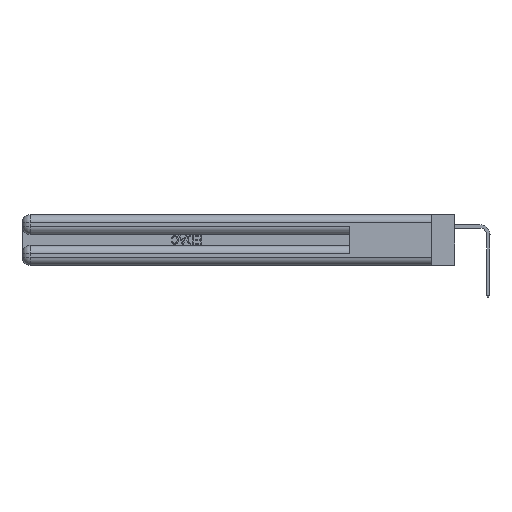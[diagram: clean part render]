
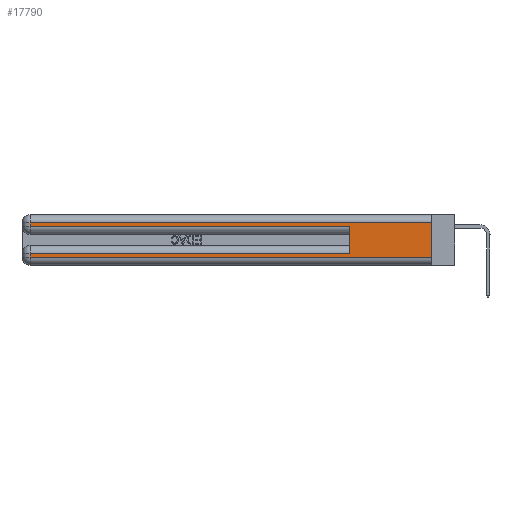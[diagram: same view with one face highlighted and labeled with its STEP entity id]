
A CAD part, left-side view. The second image highlights one B-rep face of the part: STEP entity #17790.
In plain terms, the highlighted planar face has unit normal (-1, 0, 0).
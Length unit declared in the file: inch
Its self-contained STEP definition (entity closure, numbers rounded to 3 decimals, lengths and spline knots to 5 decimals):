
#31 = DIRECTION ( 'NONE',  ( 0., 0., -1. ) ) ;
#1540 = ORIENTED_EDGE ( 'NONE', *, *, #18383, .T. ) ;
#2909 = EDGE_CURVE ( 'NONE', #14189, #25815, #42694, .T. ) ;
#3373 = DIRECTION ( 'NONE',  ( 0., 0., -1. ) ) ;
#3697 = VECTOR ( 'NONE', #49664, 39.37008 ) ;
#3704 = VECTOR ( 'NONE', #16818, 39.37008 ) ;
#4127 = EDGE_CURVE ( 'NONE', #10001, #32581, #5407, .T. ) ;
#4597 = VERTEX_POINT ( 'NONE', #41299 ) ;
#5407 = LINE ( 'NONE', #25441, #39247 ) ;
#7074 = DIRECTION ( 'NONE',  ( 0., 1., 0. ) ) ;
#7449 = CARTESIAN_POINT ( 'NONE',  ( 0., 0.6, 0.145 ) ) ;
#10001 = VERTEX_POINT ( 'NONE', #15341 ) ;
#10906 = EDGE_LOOP ( 'NONE', ( #52240, #1540, #43547, #44859, #22617, #43677, #44469, #35315 ) ) ;
#11749 = CARTESIAN_POINT ( 'NONE',  ( 0., 2.94, 0.285 ) ) ;
#14189 = VERTEX_POINT ( 'NONE', #26636 ) ;
#14384 = LINE ( 'NONE', #15727, #23009 ) ;
#15008 = LINE ( 'NONE', #36868, #3697 ) ;
#15341 = CARTESIAN_POINT ( 'NONE',  ( 0., 2.94, 0.31 ) ) ;
#15727 = CARTESIAN_POINT ( 'NONE',  ( 0., 2.94, 0.37 ) ) ;
#16026 = DIRECTION ( 'NONE',  ( 0., 0., 1. ) ) ;
#16818 = DIRECTION ( 'NONE',  ( 0., 0., -1. ) ) ;
#17790 = ADVANCED_FACE ( 'NONE', ( #39745 ), #54167, .F. ) ;
#18383 = EDGE_CURVE ( 'NONE', #41855, #10001, #15008, .T. ) ;
#19090 = CARTESIAN_POINT ( 'NONE',  ( 0., 0., 0.285 ) ) ;
#19695 = CARTESIAN_POINT ( 'NONE',  ( 0., 0.6, 0.085 ) ) ;
#19762 = VERTEX_POINT ( 'NONE', #19695 ) ;
#20041 = LINE ( 'NONE', #32479, #42573 ) ;
#20544 = VECTOR ( 'NONE', #48741, 39.37008 ) ;
#20728 = CARTESIAN_POINT ( 'NONE',  ( 0., 0., 0.06 ) ) ;
#22617 = ORIENTED_EDGE ( 'NONE', *, *, #54574, .F. ) ;
#23009 = VECTOR ( 'NONE', #49634, 39.37008 ) ;
#25441 = CARTESIAN_POINT ( 'NONE',  ( 0., 2.94, 0.37 ) ) ;
#25679 = EDGE_CURVE ( 'NONE', #50359, #14189, #14384, .T. ) ;
#25815 = VERTEX_POINT ( 'NONE', #20728 ) ;
#25864 = EDGE_CURVE ( 'NONE', #41855, #25815, #36221, .T. ) ;
#25935 = AXIS2_PLACEMENT_3D ( 'NONE', #49916, #28797, #3373 ) ;
#26636 = CARTESIAN_POINT ( 'NONE',  ( 0., 2.94, 0.06 ) ) ;
#28797 = DIRECTION ( 'NONE',  ( 1., 0., 0. ) ) ;
#30495 = LINE ( 'NONE', #19090, #20544 ) ;
#31262 = CARTESIAN_POINT ( 'NONE',  ( 0., 0., 0.06 ) ) ;
#31442 = VECTOR ( 'NONE', #48291, 39.37008 ) ;
#32479 = CARTESIAN_POINT ( 'NONE',  ( 0., 0., 0.085 ) ) ;
#32581 = VERTEX_POINT ( 'NONE', #11749 ) ;
#33129 = EDGE_CURVE ( 'NONE', #19762, #50359, #20041, .T. ) ;
#34753 = VECTOR ( 'NONE', #16026, 39.37008 ) ;
#35315 = ORIENTED_EDGE ( 'NONE', *, *, #2909, .T. ) ;
#36221 = LINE ( 'NONE', #42197, #3704 ) ;
#36481 = EDGE_CURVE ( 'NONE', #32581, #4597, #30495, .T. ) ;
#36868 = CARTESIAN_POINT ( 'NONE',  ( 0., 0., 0.31 ) ) ;
#39247 = VECTOR ( 'NONE', #31, 39.37008 ) ;
#39745 = FACE_OUTER_BOUND ( 'NONE', #10906, .T. ) ;
#41299 = CARTESIAN_POINT ( 'NONE',  ( 0., 0.6, 0.285 ) ) ;
#41855 = VERTEX_POINT ( 'NONE', #45962 ) ;
#42197 = CARTESIAN_POINT ( 'NONE',  ( 0., 0., 0.37 ) ) ;
#42573 = VECTOR ( 'NONE', #7074, 39.37008 ) ;
#42694 = LINE ( 'NONE', #31262, #31442 ) ;
#43547 = ORIENTED_EDGE ( 'NONE', *, *, #4127, .T. ) ;
#43677 = ORIENTED_EDGE ( 'NONE', *, *, #33129, .T. ) ;
#44469 = ORIENTED_EDGE ( 'NONE', *, *, #25679, .T. ) ;
#44859 = ORIENTED_EDGE ( 'NONE', *, *, #36481, .T. ) ;
#45962 = CARTESIAN_POINT ( 'NONE',  ( 0., 0., 0.31 ) ) ;
#46022 = LINE ( 'NONE', #7449, #34753 ) ;
#48291 = DIRECTION ( 'NONE',  ( 0., -1., 0. ) ) ;
#48741 = DIRECTION ( 'NONE',  ( 0., -1., 0. ) ) ;
#49532 = CARTESIAN_POINT ( 'NONE',  ( 0., 2.94, 0.085 ) ) ;
#49634 = DIRECTION ( 'NONE',  ( 0., 0., -1. ) ) ;
#49664 = DIRECTION ( 'NONE',  ( 0., 1., 0. ) ) ;
#49916 = CARTESIAN_POINT ( 'NONE',  ( 0., 0., 0.37 ) ) ;
#50359 = VERTEX_POINT ( 'NONE', #49532 ) ;
#52240 = ORIENTED_EDGE ( 'NONE', *, *, #25864, .F. ) ;
#54167 = PLANE ( 'NONE',  #25935 ) ;
#54574 = EDGE_CURVE ( 'NONE', #19762, #4597, #46022, .T. ) ;
